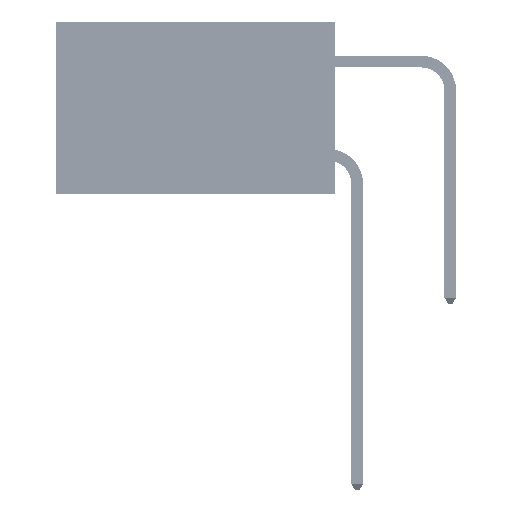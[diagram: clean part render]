
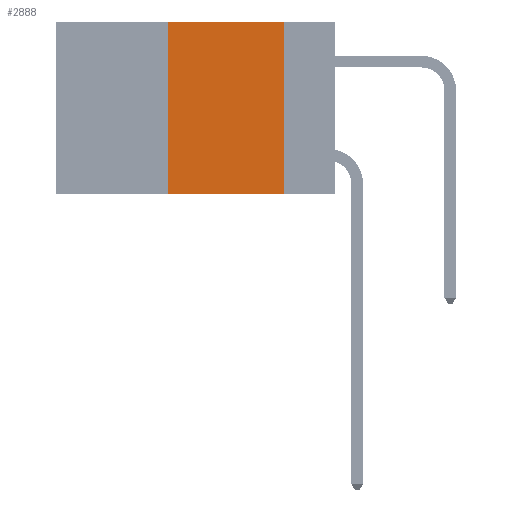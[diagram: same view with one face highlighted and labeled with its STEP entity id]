
A CAD part, left-side view. The second image highlights one B-rep face of the part: STEP entity #2888.
In plain terms, the highlighted planar face has unit normal (-1, 0, 0).
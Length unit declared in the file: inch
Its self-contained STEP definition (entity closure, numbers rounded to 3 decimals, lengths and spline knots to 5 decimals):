
#1104 = EDGE_CURVE ( 'NONE', #9755, #16856, #2529, .T. ) ;
#1919 = DIRECTION ( 'NONE',  ( 0., -1., 0. ) ) ;
#2529 = LINE ( 'NONE', #14854, #21400 ) ;
#2888 = ADVANCED_FACE ( 'NONE', ( #5975 ), #37554, .F. ) ;
#2918 = CARTESIAN_POINT ( 'NONE',  ( 0., 0.11, 0. ) ) ;
#5975 = FACE_OUTER_BOUND ( 'NONE', #7587, .T. ) ;
#6106 = CARTESIAN_POINT ( 'NONE',  ( 0., 0.6, -0.37 ) ) ;
#7405 = VECTOR ( 'NONE', #30220, 39.37008 ) ;
#7587 = EDGE_LOOP ( 'NONE', ( #32070, #21750, #40671, #46630 ) ) ;
#8247 = CARTESIAN_POINT ( 'NONE',  ( 0., 0.36, 0. ) ) ;
#8887 = EDGE_CURVE ( 'NONE', #16856, #22152, #15916, .T. ) ;
#9755 = VERTEX_POINT ( 'NONE', #13336 ) ;
#10489 = DIRECTION ( 'NONE',  ( 0., 0., -1. ) ) ;
#11738 = EDGE_CURVE ( 'NONE', #9755, #33049, #17431, .T. ) ;
#13336 = CARTESIAN_POINT ( 'NONE',  ( 0., 0.36, -0.37 ) ) ;
#14854 = CARTESIAN_POINT ( 'NONE',  ( 0., 0.36, 0. ) ) ;
#15916 = LINE ( 'NONE', #41301, #7405 ) ;
#16856 = VERTEX_POINT ( 'NONE', #8247 ) ;
#17163 = AXIS2_PLACEMENT_3D ( 'NONE', #23094, #22927, #42508 ) ;
#17431 = LINE ( 'NONE', #6106, #44811 ) ;
#17630 = CARTESIAN_POINT ( 'NONE',  ( 0., 0.11, -0.37 ) ) ;
#21400 = VECTOR ( 'NONE', #26558, 39.37008 ) ;
#21750 = ORIENTED_EDGE ( 'NONE', *, *, #8887, .F. ) ;
#22152 = VERTEX_POINT ( 'NONE', #2918 ) ;
#22927 = DIRECTION ( 'NONE',  ( 1., 0., 0. ) ) ;
#23094 = CARTESIAN_POINT ( 'NONE',  ( 0., 0.6, 0. ) ) ;
#26558 = DIRECTION ( 'NONE',  ( 0., 0., 1. ) ) ;
#28604 = VECTOR ( 'NONE', #10489, 39.37008 ) ;
#30220 = DIRECTION ( 'NONE',  ( 0., -1., 0. ) ) ;
#32070 = ORIENTED_EDGE ( 'NONE', *, *, #49829, .F. ) ;
#33049 = VERTEX_POINT ( 'NONE', #17630 ) ;
#33758 = CARTESIAN_POINT ( 'NONE',  ( 0., 0.11, 0. ) ) ;
#37554 = PLANE ( 'NONE',  #17163 ) ;
#40671 = ORIENTED_EDGE ( 'NONE', *, *, #1104, .F. ) ;
#41301 = CARTESIAN_POINT ( 'NONE',  ( 0., 0.6, 0. ) ) ;
#42508 = DIRECTION ( 'NONE',  ( 0., 0., -1. ) ) ;
#44811 = VECTOR ( 'NONE', #1919, 39.37008 ) ;
#46630 = ORIENTED_EDGE ( 'NONE', *, *, #11738, .T. ) ;
#49354 = LINE ( 'NONE', #33758, #28604 ) ;
#49829 = EDGE_CURVE ( 'NONE', #22152, #33049, #49354, .T. ) ;
